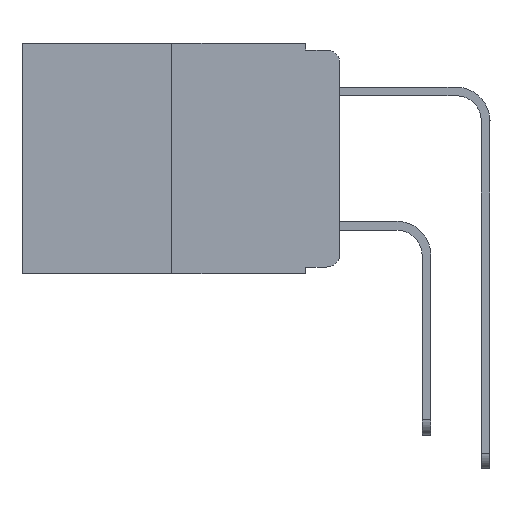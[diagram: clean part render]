
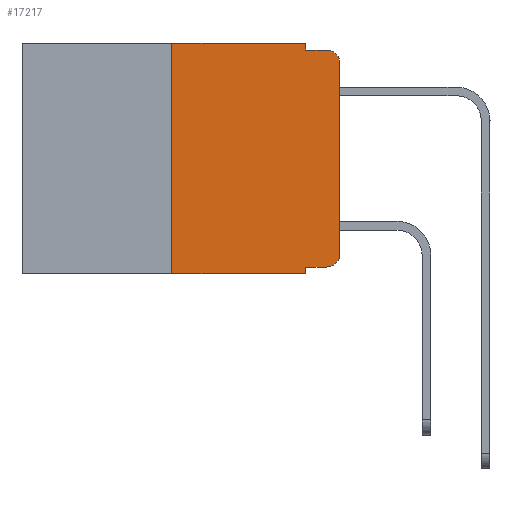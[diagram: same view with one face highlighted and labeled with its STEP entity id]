
A CAD part, left-side view. The second image highlights one B-rep face of the part: STEP entity #17217.
In plain terms, the highlighted planar face has unit normal (-1, 0, 0).
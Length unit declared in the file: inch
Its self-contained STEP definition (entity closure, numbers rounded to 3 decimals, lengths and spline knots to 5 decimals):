
#308 = VECTOR ( 'NONE', #4829, 39.37008 ) ;
#447 = ORIENTED_EDGE ( 'NONE', *, *, #17130, .F. ) ;
#662 = EDGE_CURVE ( 'NONE', #7802, #8471, #9653, .T. ) ;
#920 = CARTESIAN_POINT ( 'NONE',  ( 0., 0.051, 0. ) ) ;
#1425 = DIRECTION ( 'NONE',  ( -1., 0., 0. ) ) ;
#1695 = DIRECTION ( 'NONE',  ( 0., 0., -1. ) ) ;
#1931 = CARTESIAN_POINT ( 'NONE',  ( 0., 0.02, -0.333 ) ) ;
#2627 = VERTEX_POINT ( 'NONE', #7524 ) ;
#2867 = VERTEX_POINT ( 'NONE', #17465 ) ;
#3150 = DIRECTION ( 'NONE',  ( 0., 0., -1. ) ) ;
#3694 = EDGE_CURVE ( 'NONE', #24348, #7802, #5747, .T. ) ;
#3749 = CIRCLE ( 'NONE', #14829, 0.02 ) ;
#4204 = LINE ( 'NONE', #23972, #25833 ) ;
#4289 = VERTEX_POINT ( 'NONE', #1931 ) ;
#4598 = LINE ( 'NONE', #11552, #21475 ) ;
#4786 = DIRECTION ( 'NONE',  ( -1., 0., 0. ) ) ;
#4829 = DIRECTION ( 'NONE',  ( 0., -1., 0. ) ) ;
#4871 = CARTESIAN_POINT ( 'NONE',  ( 0., 0., -0.03 ) ) ;
#5508 = VECTOR ( 'NONE', #18591, 39.37008 ) ;
#5747 = LINE ( 'NONE', #8932, #27189 ) ;
#6260 = LINE ( 'NONE', #23649, #308 ) ;
#6854 = CARTESIAN_POINT ( 'NONE',  ( 0., 0.473, -0.343 ) ) ;
#7524 = CARTESIAN_POINT ( 'NONE',  ( 0., 0.051, 0. ) ) ;
#7583 = LINE ( 'NONE', #7617, #5508 ) ;
#7617 = CARTESIAN_POINT ( 'NONE',  ( 0., 0.473, 0. ) ) ;
#7802 = VERTEX_POINT ( 'NONE', #4871 ) ;
#8309 = PLANE ( 'NONE',  #10952 ) ;
#8471 = VERTEX_POINT ( 'NONE', #11796 ) ;
#8932 = CARTESIAN_POINT ( 'NONE',  ( 0., 0., 0. ) ) ;
#9485 = ORIENTED_EDGE ( 'NONE', *, *, #25337, .F. ) ;
#9522 = CARTESIAN_POINT ( 'NONE',  ( 0., 0.02, -0.03 ) ) ;
#9653 = CIRCLE ( 'NONE', #18542, 0.02 ) ;
#10188 = CARTESIAN_POINT ( 'NONE',  ( 0., 0.051, 0. ) ) ;
#10203 = VECTOR ( 'NONE', #25602, 39.37008 ) ;
#10548 = CARTESIAN_POINT ( 'NONE',  ( 0., 0.051, -0.343 ) ) ;
#10822 = ORIENTED_EDGE ( 'NONE', *, *, #19919, .F. ) ;
#10844 = CARTESIAN_POINT ( 'NONE',  ( 0., 0.051, -0.01 ) ) ;
#10952 = AXIS2_PLACEMENT_3D ( 'NONE', #22835, #24882, #12547 ) ;
#11012 = DIRECTION ( 'NONE',  ( 0., 0., 1. ) ) ;
#11241 = EDGE_CURVE ( 'NONE', #20321, #2627, #7583, .T. ) ;
#11519 = VECTOR ( 'NONE', #20557, 39.37008 ) ;
#11543 = EDGE_CURVE ( 'NONE', #4289, #24348, #3749, .T. ) ;
#11552 = CARTESIAN_POINT ( 'NONE',  ( 0., 0.051, -0.333 ) ) ;
#11796 = CARTESIAN_POINT ( 'NONE',  ( 0., 0.02, -0.01 ) ) ;
#12220 = CARTESIAN_POINT ( 'NONE',  ( 0., 0.25, -0.343 ) ) ;
#12547 = DIRECTION ( 'NONE',  ( 0., 0., -1. ) ) ;
#12762 = EDGE_CURVE ( 'NONE', #24064, #16521, #16397, .T. ) ;
#13735 = ORIENTED_EDGE ( 'NONE', *, *, #3694, .T. ) ;
#14317 = EDGE_CURVE ( 'NONE', #2867, #4289, #4598, .T. ) ;
#14829 = AXIS2_PLACEMENT_3D ( 'NONE', #17558, #4786, #19657 ) ;
#16397 = LINE ( 'NONE', #6854, #10203 ) ;
#16521 = VERTEX_POINT ( 'NONE', #10548 ) ;
#16998 = ORIENTED_EDGE ( 'NONE', *, *, #12762, .T. ) ;
#17130 = EDGE_CURVE ( 'NONE', #2867, #16521, #27199, .T. ) ;
#17217 = ADVANCED_FACE ( 'NONE', ( #25982 ), #8309, .F. ) ;
#17306 = CARTESIAN_POINT ( 'NONE',  ( 0., 0., -0.313 ) ) ;
#17465 = CARTESIAN_POINT ( 'NONE',  ( 0., 0.051, -0.333 ) ) ;
#17558 = CARTESIAN_POINT ( 'NONE',  ( 0., 0.02, -0.313 ) ) ;
#17953 = DIRECTION ( 'NONE',  ( 0., 0., 1. ) ) ;
#18344 = ORIENTED_EDGE ( 'NONE', *, *, #14317, .T. ) ;
#18542 = AXIS2_PLACEMENT_3D ( 'NONE', #9522, #1425, #1695 ) ;
#18591 = DIRECTION ( 'NONE',  ( 0., -1., 0. ) ) ;
#19657 = DIRECTION ( 'NONE',  ( 0., 0., -1. ) ) ;
#19919 = EDGE_CURVE ( 'NONE', #24064, #20321, #4204, .T. ) ;
#20199 = VECTOR ( 'NONE', #3150, 39.37008 ) ;
#20321 = VERTEX_POINT ( 'NONE', #21322 ) ;
#20557 = DIRECTION ( 'NONE',  ( 0., 0., -1. ) ) ;
#21200 = ORIENTED_EDGE ( 'NONE', *, *, #23956, .F. ) ;
#21322 = CARTESIAN_POINT ( 'NONE',  ( 0., 0.25, 0. ) ) ;
#21475 = VECTOR ( 'NONE', #25923, 39.37008 ) ;
#22835 = CARTESIAN_POINT ( 'NONE',  ( 0., 0.473, 0. ) ) ;
#23649 = CARTESIAN_POINT ( 'NONE',  ( 0., 0.051, -0.01 ) ) ;
#23716 = ORIENTED_EDGE ( 'NONE', *, *, #11543, .T. ) ;
#23956 = EDGE_CURVE ( 'NONE', #2627, #24298, #25580, .T. ) ;
#23972 = CARTESIAN_POINT ( 'NONE',  ( 0., 0.25, 0. ) ) ;
#24064 = VERTEX_POINT ( 'NONE', #12220 ) ;
#24087 = EDGE_LOOP ( 'NONE', ( #13735, #25307, #9485, #21200, #26560, #10822, #16998, #447, #18344, #23716 ) ) ;
#24298 = VERTEX_POINT ( 'NONE', #10844 ) ;
#24348 = VERTEX_POINT ( 'NONE', #17306 ) ;
#24882 = DIRECTION ( 'NONE',  ( 1., 0., 0. ) ) ;
#25307 = ORIENTED_EDGE ( 'NONE', *, *, #662, .T. ) ;
#25337 = EDGE_CURVE ( 'NONE', #24298, #8471, #6260, .T. ) ;
#25580 = LINE ( 'NONE', #920, #20199 ) ;
#25602 = DIRECTION ( 'NONE',  ( 0., -1., 0. ) ) ;
#25833 = VECTOR ( 'NONE', #17953, 39.37008 ) ;
#25923 = DIRECTION ( 'NONE',  ( 0., -1., 0. ) ) ;
#25982 = FACE_OUTER_BOUND ( 'NONE', #24087, .T. ) ;
#26560 = ORIENTED_EDGE ( 'NONE', *, *, #11241, .F. ) ;
#27189 = VECTOR ( 'NONE', #11012, 39.37008 ) ;
#27199 = LINE ( 'NONE', #10188, #11519 ) ;
